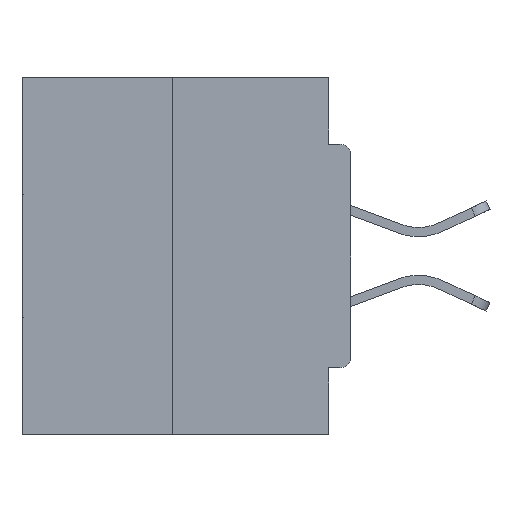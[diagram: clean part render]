
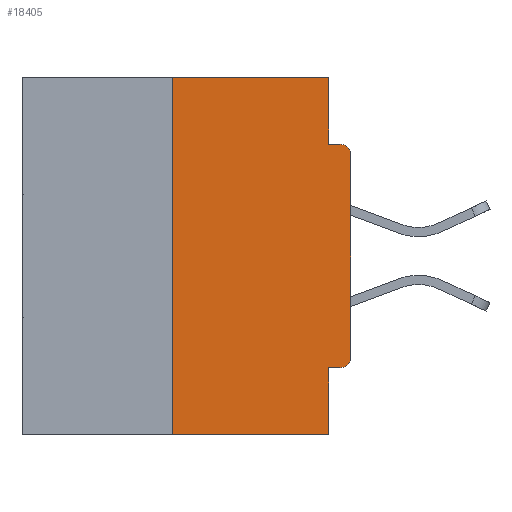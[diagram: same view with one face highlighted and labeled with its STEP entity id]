
A CAD part, left-side view. The second image highlights one B-rep face of the part: STEP entity #18405.
In plain terms, the highlighted planar face has unit normal (-1, 0, 0).
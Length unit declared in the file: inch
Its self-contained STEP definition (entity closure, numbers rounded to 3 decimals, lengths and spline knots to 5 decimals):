
#758 = AXIS2_PLACEMENT_3D ( 'NONE', #17893, #38462, #23824 ) ;
#1355 = LINE ( 'NONE', #32327, #6559 ) ;
#1842 = LINE ( 'NONE', #8970, #8935 ) ;
#2429 = CARTESIAN_POINT ( 'NONE',  ( 0., 0., -0.3915 ) ) ;
#2496 = VECTOR ( 'NONE', #16840, 39.37008 ) ;
#2878 = EDGE_CURVE ( 'NONE', #26870, #35345, #22691, .T. ) ;
#3556 = VECTOR ( 'NONE', #17755, 39.37008 ) ;
#3602 = EDGE_CURVE ( 'NONE', #33894, #19985, #10337, .T. ) ;
#3729 = ORIENTED_EDGE ( 'NONE', *, *, #3602, .T. ) ;
#4522 = DIRECTION ( 'NONE',  ( -1., 0., 0. ) ) ;
#5347 = DIRECTION ( 'NONE',  ( 0., -1., 0. ) ) ;
#5535 = CARTESIAN_POINT ( 'NONE',  ( 0., 0.031, -0.5 ) ) ;
#5819 = EDGE_CURVE ( 'NONE', #31498, #33894, #31878, .T. ) ;
#6203 = LINE ( 'NONE', #14306, #7148 ) ;
#6311 = EDGE_CURVE ( 'NONE', #17745, #19985, #6203, .T. ) ;
#6350 = CARTESIAN_POINT ( 'NONE',  ( 0., 0.015, -0.4065 ) ) ;
#6559 = VECTOR ( 'NONE', #31811, 39.37008 ) ;
#6729 = ORIENTED_EDGE ( 'NONE', *, *, #26614, .F. ) ;
#7148 = VECTOR ( 'NONE', #5347, 39.37008 ) ;
#7878 = CARTESIAN_POINT ( 'NONE',  ( 0., 0.25, 0. ) ) ;
#8098 = CARTESIAN_POINT ( 'NONE',  ( 0., 0.031, -0.4065 ) ) ;
#8115 = CARTESIAN_POINT ( 'NONE',  ( 0., 0.031, 0. ) ) ;
#8935 = VECTOR ( 'NONE', #32699, 39.37008 ) ;
#8970 = CARTESIAN_POINT ( 'NONE',  ( 0., 0.031, 0. ) ) ;
#9455 = CARTESIAN_POINT ( 'NONE',  ( 0., 0.031, -0.0935 ) ) ;
#10132 = ORIENTED_EDGE ( 'NONE', *, *, #10732, .T. ) ;
#10142 = CARTESIAN_POINT ( 'NONE',  ( 0., 0., 0. ) ) ;
#10337 = CIRCLE ( 'NONE', #758, 0.015 ) ;
#10732 = EDGE_CURVE ( 'NONE', #20020, #31498, #19592, .T. ) ;
#10747 = CARTESIAN_POINT ( 'NONE',  ( 0., 0.031, -0.5 ) ) ;
#11887 = CARTESIAN_POINT ( 'NONE',  ( 0., 0.46, -0.5 ) ) ;
#13095 = CARTESIAN_POINT ( 'NONE',  ( 0., 0.015, -0.3915 ) ) ;
#13395 = ORIENTED_EDGE ( 'NONE', *, *, #25928, .F. ) ;
#13556 = DIRECTION ( 'NONE',  ( 0., 0., 1. ) ) ;
#14306 = CARTESIAN_POINT ( 'NONE',  ( 0., 0., -0.0935 ) ) ;
#14501 = ORIENTED_EDGE ( 'NONE', *, *, #22663, .F. ) ;
#14744 = LINE ( 'NONE', #10747, #2496 ) ;
#15332 = CARTESIAN_POINT ( 'NONE',  ( 0., 0.46, 0. ) ) ;
#16840 = DIRECTION ( 'NONE',  ( 0., 0., -1. ) ) ;
#17381 = AXIS2_PLACEMENT_3D ( 'NONE', #13095, #4522, #19453 ) ;
#17745 = VERTEX_POINT ( 'NONE', #9455 ) ;
#17755 = DIRECTION ( 'NONE',  ( 0., -1., 0. ) ) ;
#17893 = CARTESIAN_POINT ( 'NONE',  ( 0., 0.015, -0.1085 ) ) ;
#18405 = ADVANCED_FACE ( 'NONE', ( #25557 ), #20840, .F. ) ;
#19261 = LINE ( 'NONE', #7878, #36161 ) ;
#19299 = VERTEX_POINT ( 'NONE', #8098 ) ;
#19453 = DIRECTION ( 'NONE',  ( 0., 0., -1. ) ) ;
#19527 = ORIENTED_EDGE ( 'NONE', *, *, #6311, .F. ) ;
#19592 = CIRCLE ( 'NONE', #17381, 0.015 ) ;
#19985 = VERTEX_POINT ( 'NONE', #27590 ) ;
#20020 = VERTEX_POINT ( 'NONE', #6350 ) ;
#20133 = VERTEX_POINT ( 'NONE', #36466 ) ;
#20317 = ORIENTED_EDGE ( 'NONE', *, *, #2878, .F. ) ;
#20636 = EDGE_CURVE ( 'NONE', #19299, #34762, #14744, .T. ) ;
#20840 = PLANE ( 'NONE',  #28811 ) ;
#21763 = ORIENTED_EDGE ( 'NONE', *, *, #5819, .T. ) ;
#22663 = EDGE_CURVE ( 'NONE', #35345, #17745, #1842, .T. ) ;
#22691 = LINE ( 'NONE', #15332, #25034 ) ;
#23824 = DIRECTION ( 'NONE',  ( 0., 0., -1. ) ) ;
#23947 = EDGE_LOOP ( 'NONE', ( #20317, #6729, #34033, #26304, #13395, #10132, #21763, #3729, #19527, #14501 ) ) ;
#24475 = DIRECTION ( 'NONE',  ( 0., -1., 0. ) ) ;
#24504 = CARTESIAN_POINT ( 'NONE',  ( 0., 0.25, 0. ) ) ;
#25034 = VECTOR ( 'NONE', #24475, 39.37008 ) ;
#25557 = FACE_OUTER_BOUND ( 'NONE', #23947, .T. ) ;
#25928 = EDGE_CURVE ( 'NONE', #20020, #19299, #1355, .T. ) ;
#26304 = ORIENTED_EDGE ( 'NONE', *, *, #20636, .F. ) ;
#26614 = EDGE_CURVE ( 'NONE', #20133, #26870, #19261, .T. ) ;
#26870 = VERTEX_POINT ( 'NONE', #24504 ) ;
#27590 = CARTESIAN_POINT ( 'NONE',  ( 0., 0.015, -0.0935 ) ) ;
#28811 = AXIS2_PLACEMENT_3D ( 'NONE', #30060, #33062, #36042 ) ;
#30060 = CARTESIAN_POINT ( 'NONE',  ( 0., 0.46, 0. ) ) ;
#31498 = VERTEX_POINT ( 'NONE', #2429 ) ;
#31811 = DIRECTION ( 'NONE',  ( 0., 1., 0. ) ) ;
#31878 = LINE ( 'NONE', #10142, #35121 ) ;
#32043 = DIRECTION ( 'NONE',  ( 0., 0., 1. ) ) ;
#32327 = CARTESIAN_POINT ( 'NONE',  ( 0., 0., -0.4065 ) ) ;
#32699 = DIRECTION ( 'NONE',  ( 0., 0., -1. ) ) ;
#33062 = DIRECTION ( 'NONE',  ( 1., 0., 0. ) ) ;
#33894 = VERTEX_POINT ( 'NONE', #33948 ) ;
#33948 = CARTESIAN_POINT ( 'NONE',  ( 0., 0., -0.1085 ) ) ;
#34033 = ORIENTED_EDGE ( 'NONE', *, *, #35977, .T. ) ;
#34762 = VERTEX_POINT ( 'NONE', #5535 ) ;
#35121 = VECTOR ( 'NONE', #13556, 39.37008 ) ;
#35193 = LINE ( 'NONE', #11887, #3556 ) ;
#35345 = VERTEX_POINT ( 'NONE', #8115 ) ;
#35977 = EDGE_CURVE ( 'NONE', #20133, #34762, #35193, .T. ) ;
#36042 = DIRECTION ( 'NONE',  ( 0., 0., -1. ) ) ;
#36161 = VECTOR ( 'NONE', #32043, 39.37008 ) ;
#36466 = CARTESIAN_POINT ( 'NONE',  ( 0., 0.25, -0.5 ) ) ;
#38462 = DIRECTION ( 'NONE',  ( -1., 0., 0. ) ) ;
